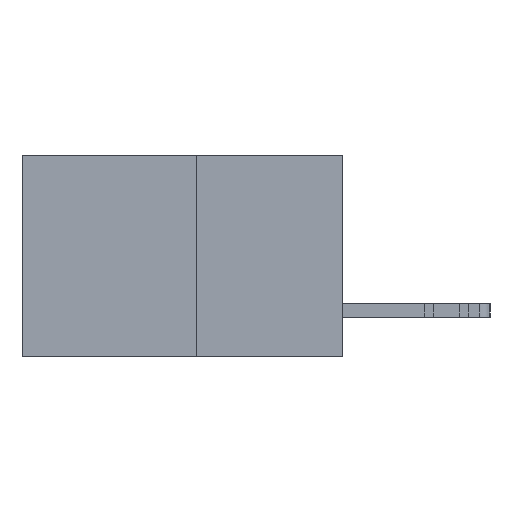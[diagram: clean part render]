
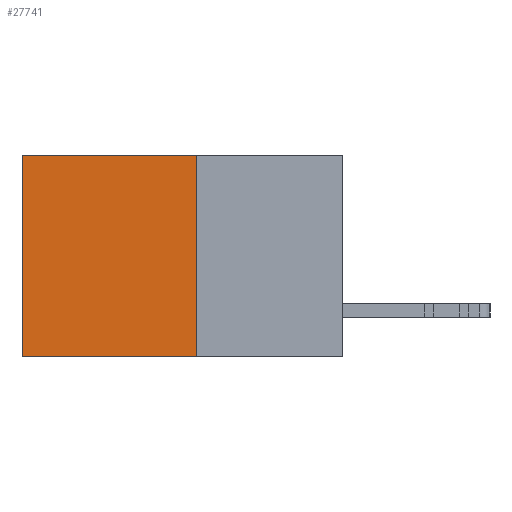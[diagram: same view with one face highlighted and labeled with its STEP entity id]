
A CAD part, left-side view. The second image highlights one B-rep face of the part: STEP entity #27741.
In plain terms, the highlighted planar face has unit normal (-1, 0, 0).
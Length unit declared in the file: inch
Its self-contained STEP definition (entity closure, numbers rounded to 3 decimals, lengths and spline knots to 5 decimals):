
#212 = CARTESIAN_POINT ( 'NONE',  ( 0.277, 0.59, 0. ) ) ;
#585 = LINE ( 'NONE', #10855, #6637 ) ;
#2150 = CARTESIAN_POINT ( 'NONE',  ( 0.277, 0.59, -0.37 ) ) ;
#2220 = VECTOR ( 'NONE', #29527, 39.37008 ) ;
#2998 = VECTOR ( 'NONE', #9951, 39.37008 ) ;
#3000 = ORIENTED_EDGE ( 'NONE', *, *, #7182, .F. ) ;
#5664 = DIRECTION ( 'NONE',  ( 0., 1., 0. ) ) ;
#6258 = CARTESIAN_POINT ( 'NONE',  ( 0.277, 0.27, 0. ) ) ;
#6637 = VECTOR ( 'NONE', #5664, 39.37008 ) ;
#6856 = VECTOR ( 'NONE', #31323, 39.37008 ) ;
#7156 = AXIS2_PLACEMENT_3D ( 'NONE', #7699, #25656, #10302 ) ;
#7182 = EDGE_CURVE ( 'NONE', #30869, #23647, #30386, .T. ) ;
#7699 = CARTESIAN_POINT ( 'NONE',  ( 0.277, 0.27, -0.37 ) ) ;
#9888 = LINE ( 'NONE', #2150, #2998 ) ;
#9951 = DIRECTION ( 'NONE',  ( 0., 0., -1. ) ) ;
#10302 = DIRECTION ( 'NONE',  ( 0., 0., -1. ) ) ;
#10855 = CARTESIAN_POINT ( 'NONE',  ( 0.277, 0.27, 0. ) ) ;
#15235 = PLANE ( 'NONE',  #7156 ) ;
#16771 = EDGE_CURVE ( 'NONE', #17265, #30869, #20481, .T. ) ;
#17265 = VERTEX_POINT ( 'NONE', #6258 ) ;
#17947 = ORIENTED_EDGE ( 'NONE', *, *, #30971, .T. ) ;
#18469 = CARTESIAN_POINT ( 'NONE',  ( 0.277, 0.27, -0.37 ) ) ;
#19841 = EDGE_CURVE ( 'NONE', #17265, #26485, #585, .T. ) ;
#20481 = LINE ( 'NONE', #18469, #6856 ) ;
#22082 = ORIENTED_EDGE ( 'NONE', *, *, #19841, .T. ) ;
#23207 = ORIENTED_EDGE ( 'NONE', *, *, #16771, .F. ) ;
#23647 = VERTEX_POINT ( 'NONE', #33158 ) ;
#25656 = DIRECTION ( 'NONE',  ( 1., 0., 0. ) ) ;
#26485 = VERTEX_POINT ( 'NONE', #212 ) ;
#27741 = ADVANCED_FACE ( 'NONE', ( #30220 ), #15235, .F. ) ;
#28082 = EDGE_LOOP ( 'NONE', ( #17947, #3000, #23207, #22082 ) ) ;
#28731 = CARTESIAN_POINT ( 'NONE',  ( 0.277, 0.27, -0.37 ) ) ;
#29527 = DIRECTION ( 'NONE',  ( 0., 1., 0. ) ) ;
#30042 = CARTESIAN_POINT ( 'NONE',  ( 0.277, 0.27, -0.37 ) ) ;
#30220 = FACE_OUTER_BOUND ( 'NONE', #28082, .T. ) ;
#30386 = LINE ( 'NONE', #28731, #2220 ) ;
#30869 = VERTEX_POINT ( 'NONE', #30042 ) ;
#30971 = EDGE_CURVE ( 'NONE', #26485, #23647, #9888, .T. ) ;
#31323 = DIRECTION ( 'NONE',  ( 0., 0., -1. ) ) ;
#33158 = CARTESIAN_POINT ( 'NONE',  ( 0.277, 0.59, -0.37 ) ) ;
